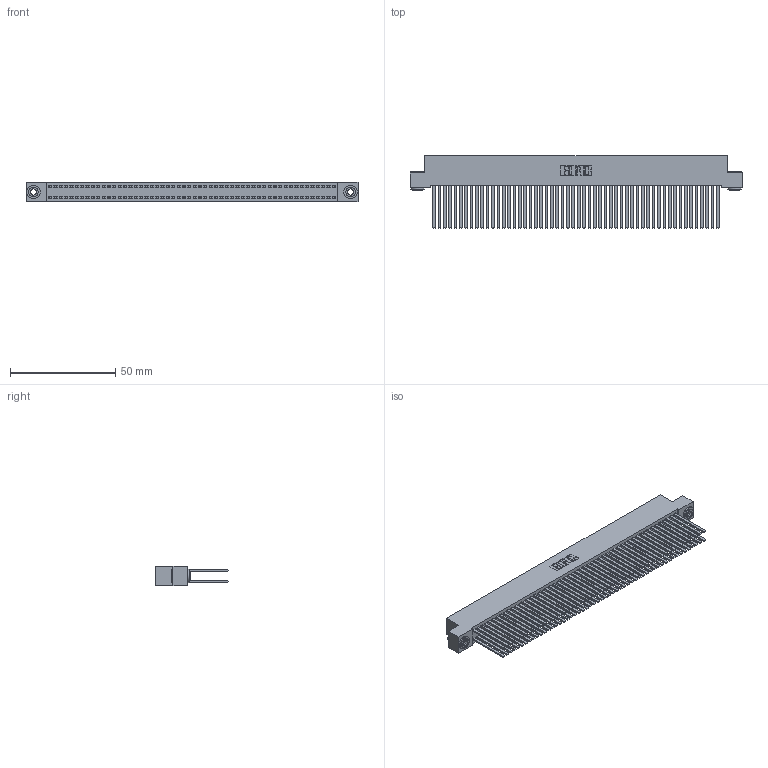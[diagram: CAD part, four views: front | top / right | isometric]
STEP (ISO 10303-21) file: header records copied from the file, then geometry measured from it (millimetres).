
FILE_DESCRIPTION (( 'STEP AP203' ), '1' );
FILE_NAME ('392-108-544-203.STEP', '2018-08-18T21:07:25', ( '' ), ( '' ), 'SwSTEP 2.0', 'SolidWorks 2016', '' );
FILE_SCHEMA (( 'CONFIG_CONTROL_DESIGN' ));
Length unit declared in the file: inch
Products named in the file (4): 342 Part_.156 TH; 345-292-001_345-293-144; 342-250-002_345-250-002-102; 392-108-544-203
Assembly tree (111 placements, depth 2):
  392-108-544-203
    342 Part_.156 TH
    345-292-001_345-293-144  x108
    342-250-002_345-250-002-102  x2
Bounding box: 157.48 x 34.3 x 9.4 mm (x, y, z)
Volume: 15743.1 mm3; surface area: 30328.3 mm2
Topology: 111 solids, 111 shells, 5116 faces, 15171 edges, 9966 vertices
Faces by surface type: plane 3532, cylinder 1576, cone 8
Entity records: 33522 total; most frequent: CARTESIAN_POINT 5513, ORIENTED_EDGE 5442, DIRECTION 4719, EDGE_CURVE 2721, LINE 2573, VECTOR 2573, VERTEX_POINT 1810, AXIS2_PLACEMENT_3D 1073
